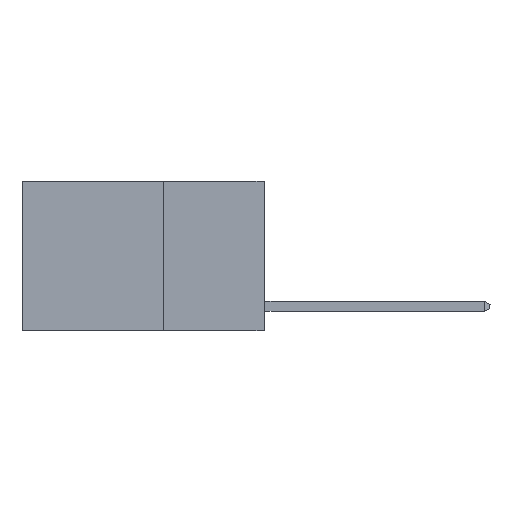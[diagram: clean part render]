
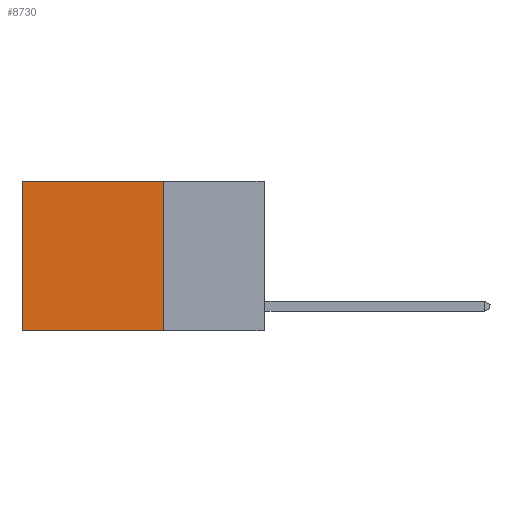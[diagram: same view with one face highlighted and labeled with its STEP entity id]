
A CAD part, left-side view. The second image highlights one B-rep face of the part: STEP entity #8730.
In plain terms, the highlighted planar face has unit normal (-1, 0, 0).
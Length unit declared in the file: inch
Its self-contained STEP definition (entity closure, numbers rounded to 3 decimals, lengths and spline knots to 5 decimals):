
#976 = CARTESIAN_POINT ( 'NONE',  ( 0.2625, 0.25, 0. ) ) ;
#2267 = VERTEX_POINT ( 'NONE', #16767 ) ;
#2395 = ORIENTED_EDGE ( 'NONE', *, *, #6545, .F. ) ;
#5210 = VERTEX_POINT ( 'NONE', #24948 ) ;
#5396 = ORIENTED_EDGE ( 'NONE', *, *, #6227, .T. ) ;
#5413 = AXIS2_PLACEMENT_3D ( 'NONE', #21165, #14736, #12332 ) ;
#6227 = EDGE_CURVE ( 'NONE', #7115, #2267, #10726, .T. ) ;
#6545 = EDGE_CURVE ( 'NONE', #5210, #8705, #21367, .T. ) ;
#7077 = VECTOR ( 'NONE', #20459, 39.37008 ) ;
#7115 = VERTEX_POINT ( 'NONE', #13732 ) ;
#7299 = ORIENTED_EDGE ( 'NONE', *, *, #12152, .F. ) ;
#7672 = ORIENTED_EDGE ( 'NONE', *, *, #27468, .T. ) ;
#8705 = VERTEX_POINT ( 'NONE', #18745 ) ;
#8730 = ADVANCED_FACE ( 'NONE', ( #13915 ), #21069, .F. ) ;
#10726 = LINE ( 'NONE', #22171, #22386 ) ;
#12152 = EDGE_CURVE ( 'NONE', #8705, #2267, #24697, .T. ) ;
#12332 = DIRECTION ( 'NONE',  ( 0., 0., -1. ) ) ;
#13673 = DIRECTION ( 'NONE',  ( 0., 1., 0. ) ) ;
#13732 = CARTESIAN_POINT ( 'NONE',  ( 0.2625, 0.6, 0. ) ) ;
#13858 = CARTESIAN_POINT ( 'NONE',  ( 0.2625, 0.25, -0.37 ) ) ;
#13915 = FACE_OUTER_BOUND ( 'NONE', #19868, .T. ) ;
#14736 = DIRECTION ( 'NONE',  ( 1., 0., 0. ) ) ;
#15315 = VECTOR ( 'NONE', #13673, 39.37008 ) ;
#15792 = DIRECTION ( 'NONE',  ( 0., 1., 0. ) ) ;
#16767 = CARTESIAN_POINT ( 'NONE',  ( 0.2625, 0.6, -0.37 ) ) ;
#18745 = CARTESIAN_POINT ( 'NONE',  ( 0.2625, 0.25, -0.37 ) ) ;
#18874 = LINE ( 'NONE', #976, #24571 ) ;
#19868 = EDGE_LOOP ( 'NONE', ( #5396, #7299, #2395, #7672 ) ) ;
#20459 = DIRECTION ( 'NONE',  ( 0., 0., -1. ) ) ;
#21069 = PLANE ( 'NONE',  #5413 ) ;
#21165 = CARTESIAN_POINT ( 'NONE',  ( 0.2625, 0.25, 0. ) ) ;
#21367 = LINE ( 'NONE', #24598, #7077 ) ;
#22171 = CARTESIAN_POINT ( 'NONE',  ( 0.2625, 0.6, 0. ) ) ;
#22386 = VECTOR ( 'NONE', #24419, 39.37008 ) ;
#24419 = DIRECTION ( 'NONE',  ( 0., 0., -1. ) ) ;
#24571 = VECTOR ( 'NONE', #15792, 39.37008 ) ;
#24598 = CARTESIAN_POINT ( 'NONE',  ( 0.2625, 0.25, 0. ) ) ;
#24697 = LINE ( 'NONE', #13858, #15315 ) ;
#24948 = CARTESIAN_POINT ( 'NONE',  ( 0.2625, 0.25, 0. ) ) ;
#27468 = EDGE_CURVE ( 'NONE', #5210, #7115, #18874, .T. ) ;
